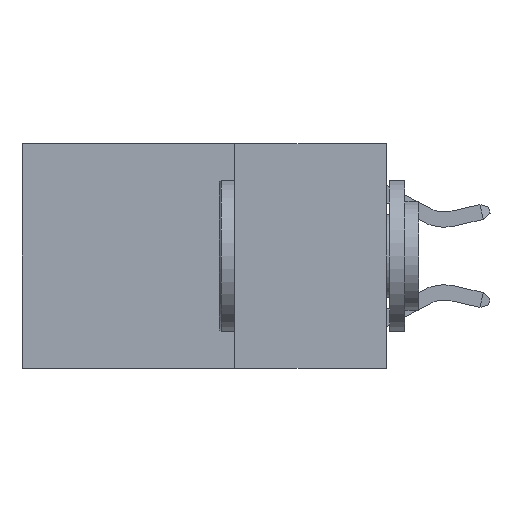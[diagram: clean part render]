
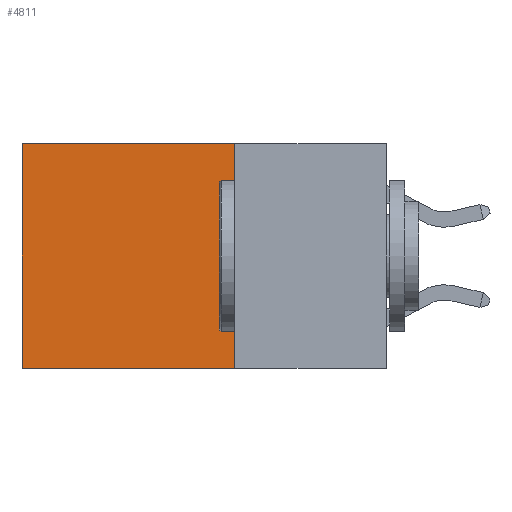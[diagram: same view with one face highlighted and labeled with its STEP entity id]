
A CAD part, left-side view. The second image highlights one B-rep face of the part: STEP entity #4811.
In plain terms, the highlighted planar face has unit normal (-1, 0, 0).
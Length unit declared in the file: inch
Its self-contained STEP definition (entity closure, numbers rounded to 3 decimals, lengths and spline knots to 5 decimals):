
#484 = ORIENTED_EDGE ( 'NONE', *, *, #10385, .T. ) ;
#1501 = CARTESIAN_POINT ( 'NONE',  ( 0.2625, 0.25, 0. ) ) ;
#1934 = EDGE_CURVE ( 'NONE', #18540, #7125, #11270, .T. ) ;
#2096 = LINE ( 'NONE', #12396, #18109 ) ;
#3061 = DIRECTION ( 'NONE',  ( 0., 0., -1. ) ) ;
#3274 = EDGE_LOOP ( 'NONE', ( #9154, #3467, #16340, #484 ) ) ;
#3467 = ORIENTED_EDGE ( 'NONE', *, *, #11703, .F. ) ;
#4811 = ADVANCED_FACE ( 'NONE', ( #17282 ), #16564, .F. ) ;
#5045 = VECTOR ( 'NONE', #5740, 39.37008 ) ;
#5688 = VERTEX_POINT ( 'NONE', #15728 ) ;
#5740 = DIRECTION ( 'NONE',  ( 0., 0., -1. ) ) ;
#6207 = DIRECTION ( 'NONE',  ( 0., 1., 0. ) ) ;
#6466 = CARTESIAN_POINT ( 'NONE',  ( 0.2625, 0.25, -0.37 ) ) ;
#6739 = CARTESIAN_POINT ( 'NONE',  ( 0.2625, 0.6, 0. ) ) ;
#6941 = VECTOR ( 'NONE', #12732, 39.37008 ) ;
#7125 = VERTEX_POINT ( 'NONE', #14316 ) ;
#7257 = CARTESIAN_POINT ( 'NONE',  ( 0.2625, 0.25, 0. ) ) ;
#8275 = CARTESIAN_POINT ( 'NONE',  ( 0.2625, 0.25, 0. ) ) ;
#8808 = DIRECTION ( 'NONE',  ( 1., 0., 0. ) ) ;
#9154 = ORIENTED_EDGE ( 'NONE', *, *, #10217, .T. ) ;
#10217 = EDGE_CURVE ( 'NONE', #11810, #5688, #17407, .T. ) ;
#10385 = EDGE_CURVE ( 'NONE', #18540, #11810, #2096, .T. ) ;
#11076 = LINE ( 'NONE', #6466, #6941 ) ;
#11270 = LINE ( 'NONE', #1501, #14933 ) ;
#11703 = EDGE_CURVE ( 'NONE', #7125, #5688, #11076, .T. ) ;
#11810 = VERTEX_POINT ( 'NONE', #6739 ) ;
#11999 = AXIS2_PLACEMENT_3D ( 'NONE', #7257, #8808, #19605 ) ;
#12396 = CARTESIAN_POINT ( 'NONE',  ( 0.2625, 0.25, 0. ) ) ;
#12732 = DIRECTION ( 'NONE',  ( 0., 1., 0. ) ) ;
#14316 = CARTESIAN_POINT ( 'NONE',  ( 0.2625, 0.25, -0.37 ) ) ;
#14933 = VECTOR ( 'NONE', #3061, 39.37008 ) ;
#15728 = CARTESIAN_POINT ( 'NONE',  ( 0.2625, 0.6, -0.37 ) ) ;
#16340 = ORIENTED_EDGE ( 'NONE', *, *, #1934, .F. ) ;
#16564 = PLANE ( 'NONE',  #11999 ) ;
#17282 = FACE_OUTER_BOUND ( 'NONE', #3274, .T. ) ;
#17407 = LINE ( 'NONE', #19652, #5045 ) ;
#18109 = VECTOR ( 'NONE', #6207, 39.37008 ) ;
#18540 = VERTEX_POINT ( 'NONE', #8275 ) ;
#19605 = DIRECTION ( 'NONE',  ( 0., 0., -1. ) ) ;
#19652 = CARTESIAN_POINT ( 'NONE',  ( 0.2625, 0.6, 0. ) ) ;
